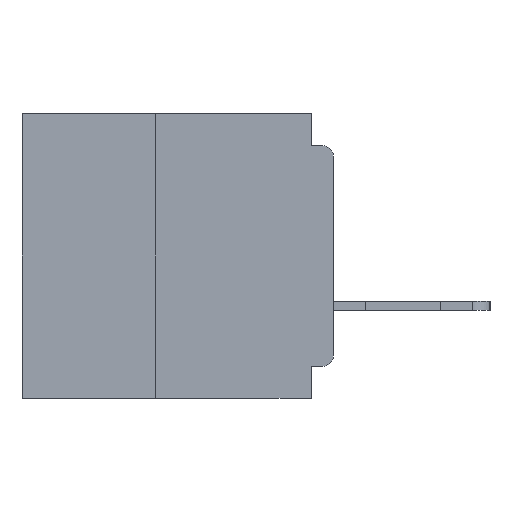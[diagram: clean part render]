
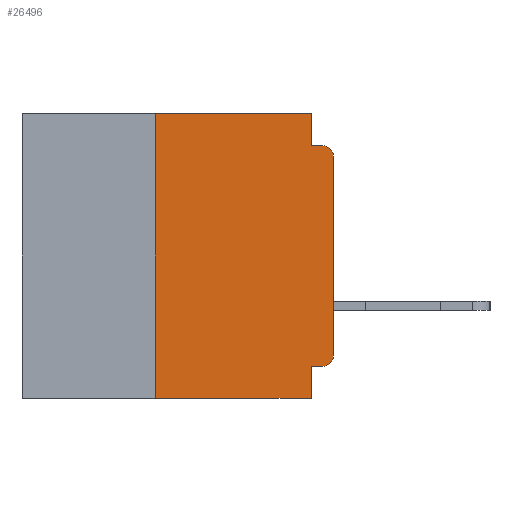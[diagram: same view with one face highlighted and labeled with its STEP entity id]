
A CAD part, left-side view. The second image highlights one B-rep face of the part: STEP entity #26496.
In plain terms, the highlighted planar face has unit normal (-1, 0, 0).
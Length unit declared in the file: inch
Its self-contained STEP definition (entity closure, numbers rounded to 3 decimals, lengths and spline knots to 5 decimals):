
#700 = ORIENTED_EDGE ( 'NONE', *, *, #35283, .T. ) ;
#1086 = CARTESIAN_POINT ( 'NONE',  ( 0., 0., -0.045 ) ) ;
#1298 = CARTESIAN_POINT ( 'NONE',  ( 0., 0.25, 0. ) ) ;
#1925 = CARTESIAN_POINT ( 'NONE',  ( 0., 0., 0. ) ) ;
#2782 = DIRECTION ( 'NONE',  ( 0., 0., -1. ) ) ;
#3313 = ORIENTED_EDGE ( 'NONE', *, *, #5218, .T. ) ;
#3359 = ORIENTED_EDGE ( 'NONE', *, *, #35579, .F. ) ;
#3726 = DIRECTION ( 'NONE',  ( 0., 0., -1. ) ) ;
#4425 = DIRECTION ( 'NONE',  ( 0., -1., 0. ) ) ;
#4432 = CARTESIAN_POINT ( 'NONE',  ( 0., 0.25, -0.4 ) ) ;
#4500 = ORIENTED_EDGE ( 'NONE', *, *, #29681, .T. ) ;
#4588 = VERTEX_POINT ( 'NONE', #5387 ) ;
#4801 = VECTOR ( 'NONE', #8972, 39.37008 ) ;
#5218 = EDGE_CURVE ( 'NONE', #4588, #43151, #28866, .T. ) ;
#5387 = CARTESIAN_POINT ( 'NONE',  ( 0., 0.015, -0.355 ) ) ;
#5518 = FACE_OUTER_BOUND ( 'NONE', #40475, .T. ) ;
#5623 = CARTESIAN_POINT ( 'NONE',  ( 0., 0.437, -0.4 ) ) ;
#5694 = LINE ( 'NONE', #15136, #22346 ) ;
#5789 = VECTOR ( 'NONE', #3726, 39.37008 ) ;
#6563 = LINE ( 'NONE', #23446, #41088 ) ;
#7120 = CARTESIAN_POINT ( 'NONE',  ( 0., 0.031, -0.4 ) ) ;
#8892 = VERTEX_POINT ( 'NONE', #12861 ) ;
#8972 = DIRECTION ( 'NONE',  ( 0., -1., 0. ) ) ;
#9099 = CARTESIAN_POINT ( 'NONE',  ( 0., 0.031, -0.355 ) ) ;
#9190 = CARTESIAN_POINT ( 'NONE',  ( 0., 0., -0.34 ) ) ;
#9279 = CARTESIAN_POINT ( 'NONE',  ( 0., 0.015, -0.34 ) ) ;
#10110 = ORIENTED_EDGE ( 'NONE', *, *, #37932, .F. ) ;
#11576 = AXIS2_PLACEMENT_3D ( 'NONE', #42831, #22722, #2782 ) ;
#12143 = DIRECTION ( 'NONE',  ( -1., 0., 0. ) ) ;
#12427 = VERTEX_POINT ( 'NONE', #20712 ) ;
#12630 = DIRECTION ( 'NONE',  ( 0., 0., -1. ) ) ;
#12861 = CARTESIAN_POINT ( 'NONE',  ( 0., 0.031, -0.4 ) ) ;
#13422 = DIRECTION ( 'NONE',  ( 0., 1., 0. ) ) ;
#14743 = LINE ( 'NONE', #4432, #30474 ) ;
#15136 = CARTESIAN_POINT ( 'NONE',  ( 0., 0.031, 0. ) ) ;
#16706 = VECTOR ( 'NONE', #40156, 39.37008 ) ;
#17207 = ORIENTED_EDGE ( 'NONE', *, *, #36887, .F. ) ;
#17523 = VERTEX_POINT ( 'NONE', #1298 ) ;
#19011 = VECTOR ( 'NONE', #38766, 39.37008 ) ;
#20712 = CARTESIAN_POINT ( 'NONE',  ( 0., 0.25, -0.4 ) ) ;
#20979 = VECTOR ( 'NONE', #4425, 39.37008 ) ;
#21421 = EDGE_CURVE ( 'NONE', #12427, #17523, #14743, .T. ) ;
#21630 = AXIS2_PLACEMENT_3D ( 'NONE', #32191, #12143, #35567 ) ;
#21823 = DIRECTION ( 'NONE',  ( 0., 0., -1. ) ) ;
#22346 = VECTOR ( 'NONE', #21823, 39.37008 ) ;
#22499 = CARTESIAN_POINT ( 'NONE',  ( 0., 0.031, -0.045 ) ) ;
#22664 = ORIENTED_EDGE ( 'NONE', *, *, #38814, .F. ) ;
#22681 = CARTESIAN_POINT ( 'NONE',  ( 0., 0.015, -0.045 ) ) ;
#22722 = DIRECTION ( 'NONE',  ( 1., 0., 0. ) ) ;
#22948 = VERTEX_POINT ( 'NONE', #32394 ) ;
#23446 = CARTESIAN_POINT ( 'NONE',  ( 0., 0., -0.355 ) ) ;
#24446 = AXIS2_PLACEMENT_3D ( 'NONE', #9279, #32696, #12630 ) ;
#24768 = ORIENTED_EDGE ( 'NONE', *, *, #37872, .F. ) ;
#25099 = ORIENTED_EDGE ( 'NONE', *, *, #27607, .T. ) ;
#25591 = LINE ( 'NONE', #26801, #16706 ) ;
#25846 = VERTEX_POINT ( 'NONE', #9099 ) ;
#26496 = ADVANCED_FACE ( 'NONE', ( #5518 ), #36116, .F. ) ;
#26801 = CARTESIAN_POINT ( 'NONE',  ( 0., 0.437, 0. ) ) ;
#27607 = EDGE_CURVE ( 'NONE', #32174, #33643, #41562, .T. ) ;
#27997 = LINE ( 'NONE', #1925, #19011 ) ;
#28866 = CIRCLE ( 'NONE', #24446, 0.015 ) ;
#29681 = EDGE_CURVE ( 'NONE', #12427, #8892, #37264, .T. ) ;
#29730 = VERTEX_POINT ( 'NONE', #22499 ) ;
#30474 = VECTOR ( 'NONE', #41289, 39.37008 ) ;
#32174 = VERTEX_POINT ( 'NONE', #41337 ) ;
#32191 = CARTESIAN_POINT ( 'NONE',  ( 0., 0.015, -0.06 ) ) ;
#32394 = CARTESIAN_POINT ( 'NONE',  ( 0., 0.031, 0. ) ) ;
#32696 = DIRECTION ( 'NONE',  ( -1., 0., 0. ) ) ;
#33534 = LINE ( 'NONE', #7120, #5789 ) ;
#33643 = VERTEX_POINT ( 'NONE', #22681 ) ;
#35283 = EDGE_CURVE ( 'NONE', #43151, #32174, #27997, .T. ) ;
#35567 = DIRECTION ( 'NONE',  ( 0., 0., -1. ) ) ;
#35579 = EDGE_CURVE ( 'NONE', #4588, #25846, #6563, .T. ) ;
#36116 = PLANE ( 'NONE',  #11576 ) ;
#36284 = ORIENTED_EDGE ( 'NONE', *, *, #21421, .F. ) ;
#36887 = EDGE_CURVE ( 'NONE', #29730, #33643, #39910, .T. ) ;
#37264 = LINE ( 'NONE', #5623, #4801 ) ;
#37872 = EDGE_CURVE ( 'NONE', #17523, #22948, #25591, .T. ) ;
#37932 = EDGE_CURVE ( 'NONE', #25846, #8892, #33534, .T. ) ;
#38766 = DIRECTION ( 'NONE',  ( 0., 0., 1. ) ) ;
#38814 = EDGE_CURVE ( 'NONE', #22948, #29730, #5694, .T. ) ;
#39910 = LINE ( 'NONE', #1086, #20979 ) ;
#40156 = DIRECTION ( 'NONE',  ( 0., -1., 0. ) ) ;
#40475 = EDGE_LOOP ( 'NONE', ( #700, #25099, #17207, #22664, #24768, #36284, #4500, #10110, #3359, #3313 ) ) ;
#41088 = VECTOR ( 'NONE', #13422, 39.37008 ) ;
#41289 = DIRECTION ( 'NONE',  ( 0., 0., 1. ) ) ;
#41337 = CARTESIAN_POINT ( 'NONE',  ( 0., 0., -0.06 ) ) ;
#41562 = CIRCLE ( 'NONE', #21630, 0.015 ) ;
#42831 = CARTESIAN_POINT ( 'NONE',  ( 0., 0.437, 0. ) ) ;
#43151 = VERTEX_POINT ( 'NONE', #9190 ) ;
